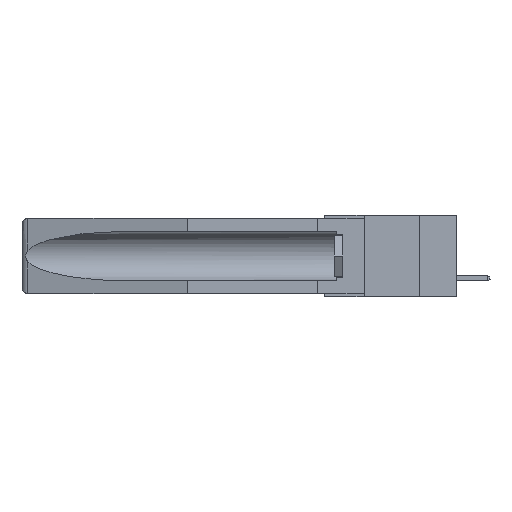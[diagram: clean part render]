
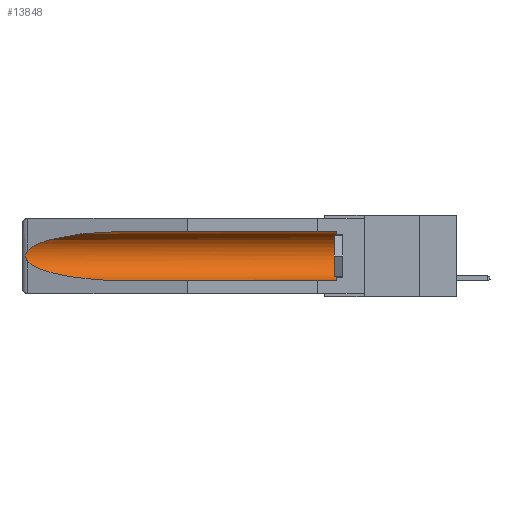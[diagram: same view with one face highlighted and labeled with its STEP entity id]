
A CAD part, left-side view. The second image highlights one B-rep face of the part: STEP entity #13848.
In plain terms, the highlighted cylindrical face has radius 2.857 mm (diameter 5.715 mm), a partial arc.
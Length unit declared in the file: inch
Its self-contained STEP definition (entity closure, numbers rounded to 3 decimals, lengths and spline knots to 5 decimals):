
#169 = CARTESIAN_POINT ( 'NONE',  ( 0.155, 1.07973, -0.059 ) ) ;
#339 = CARTESIAN_POINT ( 'NONE',  ( 0.26537, 1.52718, -0.19328 ) ) ;
#1449 = DIRECTION ( 'NONE',  ( 0., 0., 1. ) ) ;
#1757 = DIRECTION ( 'NONE',  ( 0., 1., 0. ) ) ;
#1952 = CARTESIAN_POINT ( 'NONE',  ( 0.155, -0.30754, -0.059 ) ) ;
#2086 = AXIS2_PLACEMENT_3D ( 'NONE', #19406, #10287, #1449 ) ;
#2157 = EDGE_CURVE ( 'NONE', #6476, #27332, #2420, .T. ) ;
#2420 = LINE ( 'NONE', #26439, #29144 ) ;
#3218 = FACE_OUTER_BOUND ( 'NONE', #12224, .T. ) ;
#3611 = CARTESIAN_POINT ( 'NONE',  ( 0.2673, 1.5327, -0.16383 ) ) ;
#4641 = CYLINDRICAL_SURFACE ( 'NONE', #16666, 0.1125 ) ;
#4811 = EDGE_CURVE ( 'NONE', #6476, #13599, #26445, .T. ) ;
#5966 = CARTESIAN_POINT ( 'NONE',  ( 0.2675, 1.53308, -0.17534 ) ) ;
#6118 =( BOUNDED_CURVE ( )  B_SPLINE_CURVE ( 3, ( #169, #18595, #27525, #7091 ),
 .UNSPECIFIED., .F., .F. ) 
 B_SPLINE_CURVE_WITH_KNOTS ( ( 4, 4 ),
 ( 4.71239, 6.08839 ),
 .UNSPECIFIED. ) 
 CURVE ( )  GEOMETRIC_REPRESENTATION_ITEM ( )  RATIONAL_B_SPLINE_CURVE ( ( 1., 0.848, 0.848, 1. ) ) 
 REPRESENTATION_ITEM ( '' )  );
#6308 = VERTEX_POINT ( 'NONE', #25860 ) ;
#6476 = VERTEX_POINT ( 'NONE', #19142 ) ;
#6657 = CARTESIAN_POINT ( 'NONE',  ( 0.155, 1.07973, -0.059 ) ) ;
#6857 =( BOUNDED_CURVE ( )  B_SPLINE_CURVE ( 3, ( #22734, #25425, #27461, #13977 ),
 .UNSPECIFIED., .F., .F. ) 
 B_SPLINE_CURVE_WITH_KNOTS ( ( 4, 4 ),
 ( 0.1948, 1.5708 ),
 .UNSPECIFIED. ) 
 CURVE ( )  GEOMETRIC_REPRESENTATION_ITEM ( )  RATIONAL_B_SPLINE_CURVE ( ( 1., 0.848, 0.848, 1. ) ) 
 REPRESENTATION_ITEM ( '' )  );
#6944 = CARTESIAN_POINT ( 'NONE',  ( 0.155, 0.126, -0.059 ) ) ;
#7004 = EDGE_CURVE ( 'NONE', #6308, #17357, #12178, .T. ) ;
#7091 = CARTESIAN_POINT ( 'NONE',  ( 0.26537, 1.52718, -0.14972 ) ) ;
#7822 = EDGE_CURVE ( 'NONE', #17357, #27332, #6857, .T. ) ;
#8452 = ORIENTED_EDGE ( 'NONE', *, *, #2157, .F. ) ;
#8559 = DIRECTION ( 'NONE',  ( 0., 1., 0. ) ) ;
#9785 = DIRECTION ( 'NONE',  ( 0., 0., 1. ) ) ;
#10173 = ORIENTED_EDGE ( 'NONE', *, *, #7822, .T. ) ;
#10287 = DIRECTION ( 'NONE',  ( 0., -1., 0. ) ) ;
#10376 = CARTESIAN_POINT ( 'NONE',  ( 0.26655, 1.53094, -0.18657 ) ) ;
#12178 = B_SPLINE_CURVE_WITH_KNOTS ( 'NONE', 3,
 ( #28435, #24004, #12683, #3611, #14664, #5966, #17331, #10376, #19598, #21813 ),
 .UNSPECIFIED., .F., .F.,
 ( 4, 2, 2, 2, 4 ),
 ( 0., 0.00029, 0.00058, 0.00087, 0.00117 ),
 .UNSPECIFIED. ) ;
#12224 = EDGE_LOOP ( 'NONE', ( #24251, #14688, #10173, #8452, #26941, #12513 ) ) ;
#12513 = ORIENTED_EDGE ( 'NONE', *, *, #20377, .T. ) ;
#12683 = CARTESIAN_POINT ( 'NONE',  ( 0.26654, 1.53092, -0.15636 ) ) ;
#13191 = VECTOR ( 'NONE', #8559, 39.37008 ) ;
#13599 = VERTEX_POINT ( 'NONE', #6944 ) ;
#13848 = ADVANCED_FACE ( 'NONE', ( #3218 ), #4641, .F. ) ;
#13977 = CARTESIAN_POINT ( 'NONE',  ( 0.155, 1.07973, -0.284 ) ) ;
#14664 = CARTESIAN_POINT ( 'NONE',  ( 0.2675, 1.53308, -0.16763 ) ) ;
#14688 = ORIENTED_EDGE ( 'NONE', *, *, #7004, .T. ) ;
#16666 = AXIS2_PLACEMENT_3D ( 'NONE', #16749, #23304, #9785 ) ;
#16749 = CARTESIAN_POINT ( 'NONE',  ( 0.155, -0.30754, -0.1715 ) ) ;
#17331 = CARTESIAN_POINT ( 'NONE',  ( 0.2673, 1.53269, -0.17917 ) ) ;
#17357 = VERTEX_POINT ( 'NONE', #339 ) ;
#18382 = CARTESIAN_POINT ( 'NONE',  ( 0.155, 1.07973, -0.284 ) ) ;
#18595 = CARTESIAN_POINT ( 'NONE',  ( 0.21114, 1.30732, -0.059 ) ) ;
#19142 = CARTESIAN_POINT ( 'NONE',  ( 0.155, 0.126, -0.284 ) ) ;
#19406 = CARTESIAN_POINT ( 'NONE',  ( 0.155, 0.126, -0.1715 ) ) ;
#19573 = EDGE_CURVE ( 'NONE', #24057, #6308, #6118, .T. ) ;
#19598 = CARTESIAN_POINT ( 'NONE',  ( 0.26597, 1.5296, -0.19026 ) ) ;
#20377 = EDGE_CURVE ( 'NONE', #13599, #24057, #23493, .T. ) ;
#21813 = CARTESIAN_POINT ( 'NONE',  ( 0.26537, 1.52718, -0.19328 ) ) ;
#22734 = CARTESIAN_POINT ( 'NONE',  ( 0.26537, 1.52718, -0.19328 ) ) ;
#23304 = DIRECTION ( 'NONE',  ( 0., 1., 0. ) ) ;
#23493 = LINE ( 'NONE', #1952, #13191 ) ;
#24004 = CARTESIAN_POINT ( 'NONE',  ( 0.26597, 1.52961, -0.15275 ) ) ;
#24057 = VERTEX_POINT ( 'NONE', #6657 ) ;
#24251 = ORIENTED_EDGE ( 'NONE', *, *, #19573, .T. ) ;
#25425 = CARTESIAN_POINT ( 'NONE',  ( 0.25451, 1.48313, -0.24835 ) ) ;
#25860 = CARTESIAN_POINT ( 'NONE',  ( 0.26537, 1.52718, -0.14972 ) ) ;
#26439 = CARTESIAN_POINT ( 'NONE',  ( 0.155, -0.30754, -0.284 ) ) ;
#26445 = CIRCLE ( 'NONE', #2086, 0.1125 ) ;
#26941 = ORIENTED_EDGE ( 'NONE', *, *, #4811, .T. ) ;
#27332 = VERTEX_POINT ( 'NONE', #18382 ) ;
#27461 = CARTESIAN_POINT ( 'NONE',  ( 0.21114, 1.30732, -0.284 ) ) ;
#27525 = CARTESIAN_POINT ( 'NONE',  ( 0.25451, 1.48313, -0.09465 ) ) ;
#28435 = CARTESIAN_POINT ( 'NONE',  ( 0.26537, 1.52718, -0.14972 ) ) ;
#29144 = VECTOR ( 'NONE', #1757, 39.37008 ) ;
